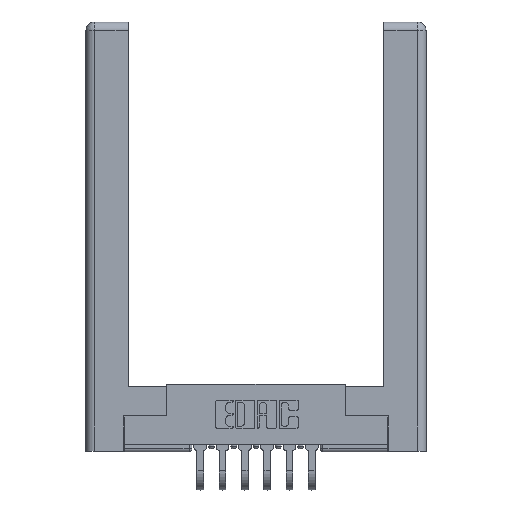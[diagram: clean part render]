
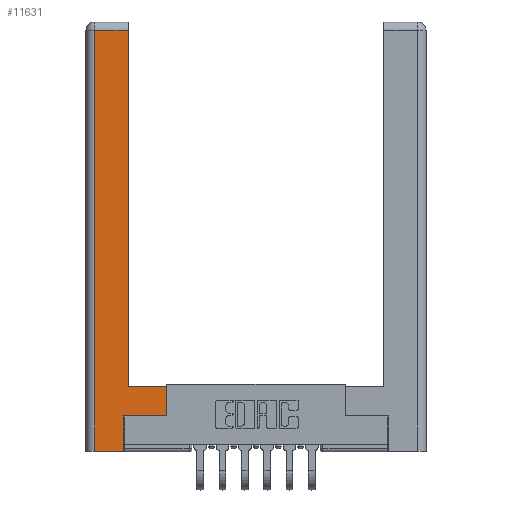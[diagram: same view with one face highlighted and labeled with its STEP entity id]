
A CAD part, top view. The second image highlights one B-rep face of the part: STEP entity #11631.
In plain terms, the highlighted planar face has unit normal (0, 0, 1).
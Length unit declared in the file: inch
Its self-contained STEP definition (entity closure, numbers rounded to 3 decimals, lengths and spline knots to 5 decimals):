
#88 = CARTESIAN_POINT ( 'NONE',  ( 0.0615, 2.94, 0. ) ) ;
#105 = DIRECTION ( 'NONE',  ( 1., 0., 0. ) ) ;
#260 = CARTESIAN_POINT ( 'NONE',  ( 0.0615, 0., 0. ) ) ;
#741 = LINE ( 'NONE', #3435, #11988 ) ;
#806 = EDGE_CURVE ( 'NONE', #1197, #11295, #7165, .T. ) ;
#1104 = EDGE_CURVE ( 'NONE', #1157, #4465, #11966, .T. ) ;
#1157 = VERTEX_POINT ( 'NONE', #5344 ) ;
#1197 = VERTEX_POINT ( 'NONE', #9097 ) ;
#1825 = CARTESIAN_POINT ( 'NONE',  ( 0.0615, 0., 0. ) ) ;
#2017 = EDGE_CURVE ( 'NONE', #8763, #1157, #741, .T. ) ;
#2043 = EDGE_CURVE ( 'NONE', #11295, #8158, #8239, .T. ) ;
#2316 = PLANE ( 'NONE',  #8939 ) ;
#2318 = VECTOR ( 'NONE', #7345, 39.37008 ) ;
#2385 = CARTESIAN_POINT ( 'NONE',  ( 0.295, 0.45, 0. ) ) ;
#2600 = ORIENTED_EDGE ( 'NONE', *, *, #3945, .T. ) ;
#3435 = CARTESIAN_POINT ( 'NONE',  ( 0.295, 3., 0. ) ) ;
#3566 = CARTESIAN_POINT ( 'NONE',  ( 0.565, 0.245, 0. ) ) ;
#3818 = ORIENTED_EDGE ( 'NONE', *, *, #8430, .T. ) ;
#3834 = ORIENTED_EDGE ( 'NONE', *, *, #1104, .T. ) ;
#3945 = EDGE_CURVE ( 'NONE', #4406, #7350, #7645, .T. ) ;
#4045 = CARTESIAN_POINT ( 'NONE',  ( 0.265, 0., 0. ) ) ;
#4144 = FACE_OUTER_BOUND ( 'NONE', #11526, .T. ) ;
#4350 = CARTESIAN_POINT ( 'NONE',  ( 0.565, 0.45, 0. ) ) ;
#4406 = VERTEX_POINT ( 'NONE', #1825 ) ;
#4437 = DIRECTION ( 'NONE',  ( 0., 1., 0. ) ) ;
#4465 = VERTEX_POINT ( 'NONE', #88 ) ;
#4728 = CARTESIAN_POINT ( 'NONE',  ( 0.265, 0., 0. ) ) ;
#4811 = CARTESIAN_POINT ( 'NONE',  ( 0.295, 0.45, 0. ) ) ;
#5178 = DIRECTION ( 'NONE',  ( -1., 0., 0. ) ) ;
#5344 = CARTESIAN_POINT ( 'NONE',  ( 0.295, 2.94, 0. ) ) ;
#5499 = VECTOR ( 'NONE', #10062, 39.37008 ) ;
#5566 = EDGE_CURVE ( 'NONE', #8158, #8763, #10963, .T. ) ;
#6121 = CARTESIAN_POINT ( 'NONE',  ( 0., 0., 0. ) ) ;
#6126 = LINE ( 'NONE', #260, #8683 ) ;
#6249 = CARTESIAN_POINT ( 'NONE',  ( 0.265, 0.245, 0. ) ) ;
#6380 = DIRECTION ( 'NONE',  ( 0., 1., 0. ) ) ;
#7165 = LINE ( 'NONE', #3566, #5499 ) ;
#7327 = LINE ( 'NONE', #6249, #7473 ) ;
#7345 = DIRECTION ( 'NONE',  ( -1., 0., 0. ) ) ;
#7350 = VERTEX_POINT ( 'NONE', #4045 ) ;
#7473 = VECTOR ( 'NONE', #6380, 39.37008 ) ;
#7645 = LINE ( 'NONE', #4728, #8506 ) ;
#7939 = DIRECTION ( 'NONE',  ( 0., 0., -1. ) ) ;
#8067 = DIRECTION ( 'NONE',  ( 0., -1., 0. ) ) ;
#8123 = EDGE_CURVE ( 'NONE', #7350, #1197, #7327, .T. ) ;
#8158 = VERTEX_POINT ( 'NONE', #4350 ) ;
#8239 = LINE ( 'NONE', #9244, #10620 ) ;
#8430 = EDGE_CURVE ( 'NONE', #4465, #4406, #6126, .T. ) ;
#8506 = VECTOR ( 'NONE', #105, 39.37008 ) ;
#8683 = VECTOR ( 'NONE', #8067, 39.37008 ) ;
#8763 = VERTEX_POINT ( 'NONE', #4811 ) ;
#8814 = VECTOR ( 'NONE', #9064, 39.37008 ) ;
#8833 = ORIENTED_EDGE ( 'NONE', *, *, #2017, .T. ) ;
#8939 = AXIS2_PLACEMENT_3D ( 'NONE', #6121, #7939, #5178 ) ;
#9064 = DIRECTION ( 'NONE',  ( -1., 0., 0. ) ) ;
#9097 = CARTESIAN_POINT ( 'NONE',  ( 0.265, 0.245, 0. ) ) ;
#9121 = DIRECTION ( 'NONE',  ( 0., 1., 0. ) ) ;
#9226 = ORIENTED_EDGE ( 'NONE', *, *, #806, .T. ) ;
#9244 = CARTESIAN_POINT ( 'NONE',  ( 0.565, 0.45, 0. ) ) ;
#9444 = ORIENTED_EDGE ( 'NONE', *, *, #8123, .T. ) ;
#9605 = ORIENTED_EDGE ( 'NONE', *, *, #2043, .T. ) ;
#9640 = CARTESIAN_POINT ( 'NONE',  ( 0.565, 0.245, 0. ) ) ;
#10062 = DIRECTION ( 'NONE',  ( 1., 0., 0. ) ) ;
#10620 = VECTOR ( 'NONE', #9121, 39.37008 ) ;
#10836 = ORIENTED_EDGE ( 'NONE', *, *, #5566, .T. ) ;
#10963 = LINE ( 'NONE', #2385, #8814 ) ;
#11295 = VERTEX_POINT ( 'NONE', #9640 ) ;
#11526 = EDGE_LOOP ( 'NONE', ( #8833, #3834, #3818, #2600, #9444, #9226, #9605, #10836 ) ) ;
#11631 = ADVANCED_FACE ( 'NONE', ( #4144 ), #2316, .F. ) ;
#11966 = LINE ( 'NONE', #12094, #2318 ) ;
#11988 = VECTOR ( 'NONE', #4437, 39.37008 ) ;
#12094 = CARTESIAN_POINT ( 'NONE',  ( 0.0615, 2.94, 0. ) ) ;
